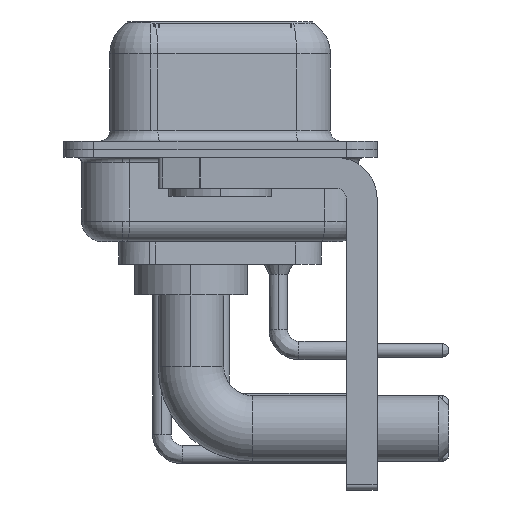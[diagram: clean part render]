
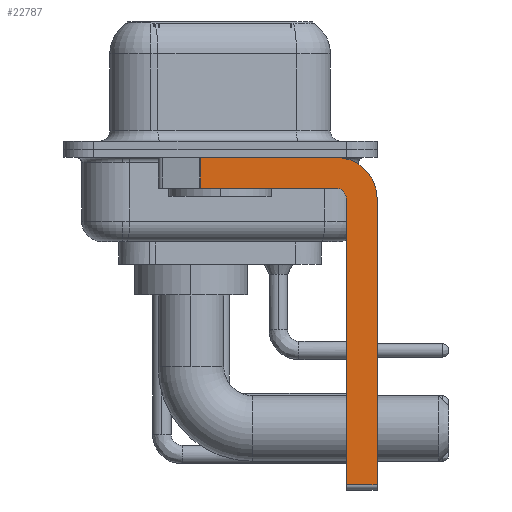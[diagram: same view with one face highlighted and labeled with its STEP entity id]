
A CAD part, left-side view. The second image highlights one B-rep face of the part: STEP entity #22787.
In plain terms, the highlighted planar face has unit normal (-1, 0, 0).
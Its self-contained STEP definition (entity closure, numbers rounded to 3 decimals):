
#836 = DIRECTION ( 'NONE',  ( 0., 0., -1. ) ) ;
#894 = DIRECTION ( 'NONE',  ( 1., 0., 0. ) ) ;
#2470 = CIRCLE ( 'NONE', #4599, 0.5 ) ;
#3093 = DIRECTION ( 'NONE',  ( 0., 0., -1. ) ) ;
#3178 = EDGE_CURVE ( 'NONE', #17456, #15104, #20879, .T. ) ;
#3188 = CARTESIAN_POINT ( 'NONE',  ( -2.9, 0.978, -1.9 ) ) ;
#3421 = CARTESIAN_POINT ( 'NONE',  ( -2.9, -5.65, -2.4 ) ) ;
#3523 = DIRECTION ( 'NONE',  ( 0., 0., 1. ) ) ;
#3682 = LINE ( 'NONE', #26446, #5216 ) ;
#4552 = ORIENTED_EDGE ( 'NONE', *, *, #3178, .F. ) ;
#4599 = AXIS2_PLACEMENT_3D ( 'NONE', #4970, #17420, #27715 ) ;
#4970 = CARTESIAN_POINT ( 'NONE',  ( -2.9, -5.65, -2.4 ) ) ;
#5216 = VECTOR ( 'NONE', #836, 1000. ) ;
#5247 = DIRECTION ( 'NONE',  ( 0., -1., 0. ) ) ;
#8111 = CARTESIAN_POINT ( 'NONE',  ( -2.9, -5.65, -1.9 ) ) ;
#8438 = CARTESIAN_POINT ( 'NONE',  ( -2.9, -6.15, -16.6 ) ) ;
#8446 = VERTEX_POINT ( 'NONE', #22425 ) ;
#8503 = EDGE_CURVE ( 'NONE', #23497, #12045, #9966, .T. ) ;
#8645 = VECTOR ( 'NONE', #3523, 1000. ) ;
#8937 = ORIENTED_EDGE ( 'NONE', *, *, #31135, .F. ) ;
#9787 = CARTESIAN_POINT ( 'NONE',  ( -2.9, -7.65, -16.35 ) ) ;
#9966 = LINE ( 'NONE', #19918, #32992 ) ;
#12045 = VERTEX_POINT ( 'NONE', #9787 ) ;
#12515 = ORIENTED_EDGE ( 'NONE', *, *, #21359, .F. ) ;
#13326 = LINE ( 'NONE', #15840, #26750 ) ;
#13526 = FACE_OUTER_BOUND ( 'NONE', #29169, .T. ) ;
#14310 = CIRCLE ( 'NONE', #31527, 2. ) ;
#14851 = VERTEX_POINT ( 'NONE', #17231 ) ;
#15104 = VERTEX_POINT ( 'NONE', #3188 ) ;
#15840 = CARTESIAN_POINT ( 'NONE',  ( -2.9, 3., -0.4 ) ) ;
#17231 = CARTESIAN_POINT ( 'NONE',  ( -2.9, -5.65, -0.4 ) ) ;
#17420 = DIRECTION ( 'NONE',  ( -1., 0., 0. ) ) ;
#17456 = VERTEX_POINT ( 'NONE', #30047 ) ;
#18412 = DIRECTION ( 'NONE',  ( 1., 0., 0. ) ) ;
#19379 = ORIENTED_EDGE ( 'NONE', *, *, #24348, .F. ) ;
#19452 = EDGE_CURVE ( 'NONE', #26519, #15104, #19489, .T. ) ;
#19489 = LINE ( 'NONE', #32126, #27765 ) ;
#19918 = CARTESIAN_POINT ( 'NONE',  ( -2.9, -5.65, -16.35 ) ) ;
#20131 = EDGE_CURVE ( 'NONE', #14851, #22512, #14310, .T. ) ;
#20879 = LINE ( 'NONE', #8111, #26790 ) ;
#21359 = EDGE_CURVE ( 'NONE', #8446, #17456, #2470, .T. ) ;
#21414 = PLANE ( 'NONE',  #22314 ) ;
#22314 = AXIS2_PLACEMENT_3D ( 'NONE', #32204, #894, #29196 ) ;
#22425 = CARTESIAN_POINT ( 'NONE',  ( -2.9, -6.15, -2.4 ) ) ;
#22456 = CARTESIAN_POINT ( 'NONE',  ( -2.9, -7.65, -2.4 ) ) ;
#22512 = VERTEX_POINT ( 'NONE', #22456 ) ;
#22787 = ADVANCED_FACE ( 'NONE', ( #13526 ), #21414, .F. ) ;
#23497 = VERTEX_POINT ( 'NONE', #30638 ) ;
#24348 = EDGE_CURVE ( 'NONE', #26519, #14851, #13326, .T. ) ;
#24911 = ORIENTED_EDGE ( 'NONE', *, *, #19452, .T. ) ;
#26001 = CARTESIAN_POINT ( 'NONE',  ( -2.9, 0.978, -0.4 ) ) ;
#26286 = DIRECTION ( 'NONE',  ( 0., 1., 0. ) ) ;
#26446 = CARTESIAN_POINT ( 'NONE',  ( -2.9, -7.65, -2.4 ) ) ;
#26519 = VERTEX_POINT ( 'NONE', #26001 ) ;
#26750 = VECTOR ( 'NONE', #5247, 1000. ) ;
#26790 = VECTOR ( 'NONE', #26286, 1000. ) ;
#27097 = EDGE_CURVE ( 'NONE', #23497, #8446, #31344, .T. ) ;
#27715 = DIRECTION ( 'NONE',  ( 0., 0., 1. ) ) ;
#27765 = VECTOR ( 'NONE', #29771, 1000. ) ;
#28017 = DIRECTION ( 'NONE',  ( 0., -1., 0. ) ) ;
#29169 = EDGE_LOOP ( 'NONE', ( #19379, #24911, #4552, #12515, #32140, #31579, #8937, #32469 ) ) ;
#29196 = DIRECTION ( 'NONE',  ( 0., 0., -1. ) ) ;
#29771 = DIRECTION ( 'NONE',  ( 0., 0., -1. ) ) ;
#30047 = CARTESIAN_POINT ( 'NONE',  ( -2.9, -5.65, -1.9 ) ) ;
#30638 = CARTESIAN_POINT ( 'NONE',  ( -2.9, -6.15, -16.35 ) ) ;
#31135 = EDGE_CURVE ( 'NONE', #22512, #12045, #3682, .T. ) ;
#31344 = LINE ( 'NONE', #8438, #8645 ) ;
#31527 = AXIS2_PLACEMENT_3D ( 'NONE', #3421, #18412, #3093 ) ;
#31579 = ORIENTED_EDGE ( 'NONE', *, *, #8503, .T. ) ;
#32126 = CARTESIAN_POINT ( 'NONE',  ( -2.9, 0.978, -1.9 ) ) ;
#32140 = ORIENTED_EDGE ( 'NONE', *, *, #27097, .F. ) ;
#32204 = CARTESIAN_POINT ( 'NONE',  ( -2.9, -5.65, -2.4 ) ) ;
#32469 = ORIENTED_EDGE ( 'NONE', *, *, #20131, .F. ) ;
#32992 = VECTOR ( 'NONE', #28017, 1000. ) ;
